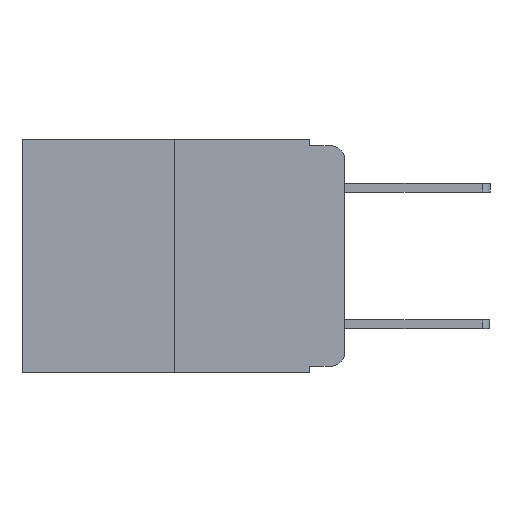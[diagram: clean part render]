
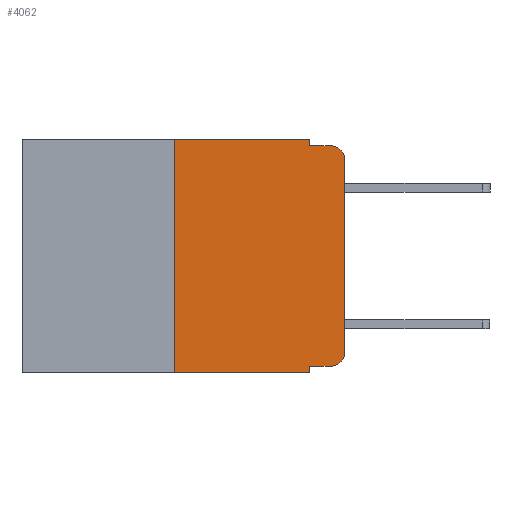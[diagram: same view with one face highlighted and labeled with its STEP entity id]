
A CAD part, left-side view. The second image highlights one B-rep face of the part: STEP entity #4062.
In plain terms, the highlighted planar face has unit normal (-1, 0, 0).
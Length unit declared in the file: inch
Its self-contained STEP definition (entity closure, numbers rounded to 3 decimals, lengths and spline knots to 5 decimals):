
#255 = CARTESIAN_POINT ( 'NONE',  ( 0., 0.051, -0.343 ) ) ;
#492 = CARTESIAN_POINT ( 'NONE',  ( 0., 0.051, 0. ) ) ;
#672 = LINE ( 'NONE', #6236, #13979 ) ;
#1037 = CARTESIAN_POINT ( 'NONE',  ( 0., 0.25, 0. ) ) ;
#1307 = EDGE_CURVE ( 'NONE', #4608, #13476, #12834, .T. ) ;
#1324 = CARTESIAN_POINT ( 'NONE',  ( 0., 0.02, -0.313 ) ) ;
#1428 = DIRECTION ( 'NONE',  ( 0., -1., 0. ) ) ;
#1768 = ORIENTED_EDGE ( 'NONE', *, *, #15326, .F. ) ;
#1850 = CIRCLE ( 'NONE', #8437, 0.02 ) ;
#1852 = VERTEX_POINT ( 'NONE', #255 ) ;
#2150 = CARTESIAN_POINT ( 'NONE',  ( 0., 0.051, -0.01 ) ) ;
#2246 = VECTOR ( 'NONE', #5467, 39.37008 ) ;
#2269 = CARTESIAN_POINT ( 'NONE',  ( 0., 0., 0. ) ) ;
#2465 = ORIENTED_EDGE ( 'NONE', *, *, #3217, .F. ) ;
#2760 = DIRECTION ( 'NONE',  ( 0., 0., -1. ) ) ;
#2817 = CARTESIAN_POINT ( 'NONE',  ( 0., 0.051, -0.333 ) ) ;
#3217 = EDGE_CURVE ( 'NONE', #7695, #6763, #15721, .T. ) ;
#3538 = AXIS2_PLACEMENT_3D ( 'NONE', #15129, #7724, #16343 ) ;
#3802 = ORIENTED_EDGE ( 'NONE', *, *, #10863, .T. ) ;
#4062 = ADVANCED_FACE ( 'NONE', ( #4171 ), #5894, .F. ) ;
#4074 = CARTESIAN_POINT ( 'NONE',  ( 0., 0.473, 0. ) ) ;
#4171 = FACE_OUTER_BOUND ( 'NONE', #7964, .T. ) ;
#4434 = ORIENTED_EDGE ( 'NONE', *, *, #1307, .F. ) ;
#4608 = VERTEX_POINT ( 'NONE', #10670 ) ;
#4694 = CARTESIAN_POINT ( 'NONE',  ( 0., 0.051, 0. ) ) ;
#4772 = LINE ( 'NONE', #2817, #14275 ) ;
#5162 = VERTEX_POINT ( 'NONE', #7065 ) ;
#5396 = CARTESIAN_POINT ( 'NONE',  ( 0., 0.02, -0.333 ) ) ;
#5444 = DIRECTION ( 'NONE',  ( 0., -1., 0. ) ) ;
#5467 = DIRECTION ( 'NONE',  ( 0., 0., 1. ) ) ;
#5894 = PLANE ( 'NONE',  #15864 ) ;
#6236 = CARTESIAN_POINT ( 'NONE',  ( 0., 0.051, -0.01 ) ) ;
#6317 = DIRECTION ( 'NONE',  ( 0., 0., 1. ) ) ;
#6464 = VECTOR ( 'NONE', #6317, 39.37008 ) ;
#6763 = VERTEX_POINT ( 'NONE', #1037 ) ;
#7065 = CARTESIAN_POINT ( 'NONE',  ( 0., 0., -0.03 ) ) ;
#7121 = CARTESIAN_POINT ( 'NONE',  ( 0., 0.473, 0. ) ) ;
#7177 = DIRECTION ( 'NONE',  ( 0., 0., -1. ) ) ;
#7237 = DIRECTION ( 'NONE',  ( 0., 0., -1. ) ) ;
#7366 = DIRECTION ( 'NONE',  ( 0., -1., 0. ) ) ;
#7571 = EDGE_CURVE ( 'NONE', #10394, #1852, #15971, .T. ) ;
#7695 = VERTEX_POINT ( 'NONE', #16025 ) ;
#7724 = DIRECTION ( 'NONE',  ( -1., 0., 0. ) ) ;
#7799 = ORIENTED_EDGE ( 'NONE', *, *, #10011, .F. ) ;
#7963 = ORIENTED_EDGE ( 'NONE', *, *, #11993, .T. ) ;
#7964 = EDGE_LOOP ( 'NONE', ( #7963, #11633, #1768, #4434, #7799, #2465, #12611, #9706, #12999, #3802 ) ) ;
#8210 = CARTESIAN_POINT ( 'NONE',  ( 0., 0.02, -0.01 ) ) ;
#8248 = VERTEX_POINT ( 'NONE', #8210 ) ;
#8437 = AXIS2_PLACEMENT_3D ( 'NONE', #1324, #10414, #2760 ) ;
#8480 = CARTESIAN_POINT ( 'NONE',  ( 0., 0.051, -0.333 ) ) ;
#9083 = EDGE_CURVE ( 'NONE', #7695, #1852, #15816, .T. ) ;
#9191 = EDGE_CURVE ( 'NONE', #10394, #9969, #4772, .T. ) ;
#9685 = DIRECTION ( 'NONE',  ( 0., 0., -1. ) ) ;
#9706 = ORIENTED_EDGE ( 'NONE', *, *, #7571, .F. ) ;
#9729 = LINE ( 'NONE', #2269, #6464 ) ;
#9969 = VERTEX_POINT ( 'NONE', #5396 ) ;
#10011 = EDGE_CURVE ( 'NONE', #6763, #4608, #11534, .T. ) ;
#10394 = VERTEX_POINT ( 'NONE', #8480 ) ;
#10414 = DIRECTION ( 'NONE',  ( -1., 0., 0. ) ) ;
#10670 = CARTESIAN_POINT ( 'NONE',  ( 0., 0.051, 0. ) ) ;
#10863 = EDGE_CURVE ( 'NONE', #9969, #14183, #1850, .T. ) ;
#11534 = LINE ( 'NONE', #4074, #14437 ) ;
#11633 = ORIENTED_EDGE ( 'NONE', *, *, #12822, .T. ) ;
#11993 = EDGE_CURVE ( 'NONE', #14183, #5162, #9729, .T. ) ;
#12253 = CARTESIAN_POINT ( 'NONE',  ( 0., 0.473, -0.343 ) ) ;
#12443 = DIRECTION ( 'NONE',  ( 0., -1., 0. ) ) ;
#12522 = VECTOR ( 'NONE', #7366, 39.37008 ) ;
#12611 = ORIENTED_EDGE ( 'NONE', *, *, #9083, .T. ) ;
#12666 = VECTOR ( 'NONE', #7237, 39.37008 ) ;
#12822 = EDGE_CURVE ( 'NONE', #5162, #8248, #15717, .T. ) ;
#12834 = LINE ( 'NONE', #492, #15748 ) ;
#12999 = ORIENTED_EDGE ( 'NONE', *, *, #9191, .T. ) ;
#13476 = VERTEX_POINT ( 'NONE', #2150 ) ;
#13505 = CARTESIAN_POINT ( 'NONE',  ( 0., 0., -0.313 ) ) ;
#13979 = VECTOR ( 'NONE', #12443, 39.37008 ) ;
#14143 = CARTESIAN_POINT ( 'NONE',  ( 0., 0.25, 0. ) ) ;
#14183 = VERTEX_POINT ( 'NONE', #13505 ) ;
#14275 = VECTOR ( 'NONE', #1428, 39.37008 ) ;
#14437 = VECTOR ( 'NONE', #5444, 39.37008 ) ;
#14573 = DIRECTION ( 'NONE',  ( 1., 0., 0. ) ) ;
#15129 = CARTESIAN_POINT ( 'NONE',  ( 0., 0.02, -0.03 ) ) ;
#15326 = EDGE_CURVE ( 'NONE', #13476, #8248, #672, .T. ) ;
#15717 = CIRCLE ( 'NONE', #3538, 0.02 ) ;
#15721 = LINE ( 'NONE', #14143, #2246 ) ;
#15748 = VECTOR ( 'NONE', #9685, 39.37008 ) ;
#15816 = LINE ( 'NONE', #12253, #12522 ) ;
#15864 = AXIS2_PLACEMENT_3D ( 'NONE', #7121, #14573, #7177 ) ;
#15971 = LINE ( 'NONE', #4694, #12666 ) ;
#16025 = CARTESIAN_POINT ( 'NONE',  ( 0., 0.25, -0.343 ) ) ;
#16343 = DIRECTION ( 'NONE',  ( 0., 0., -1. ) ) ;
